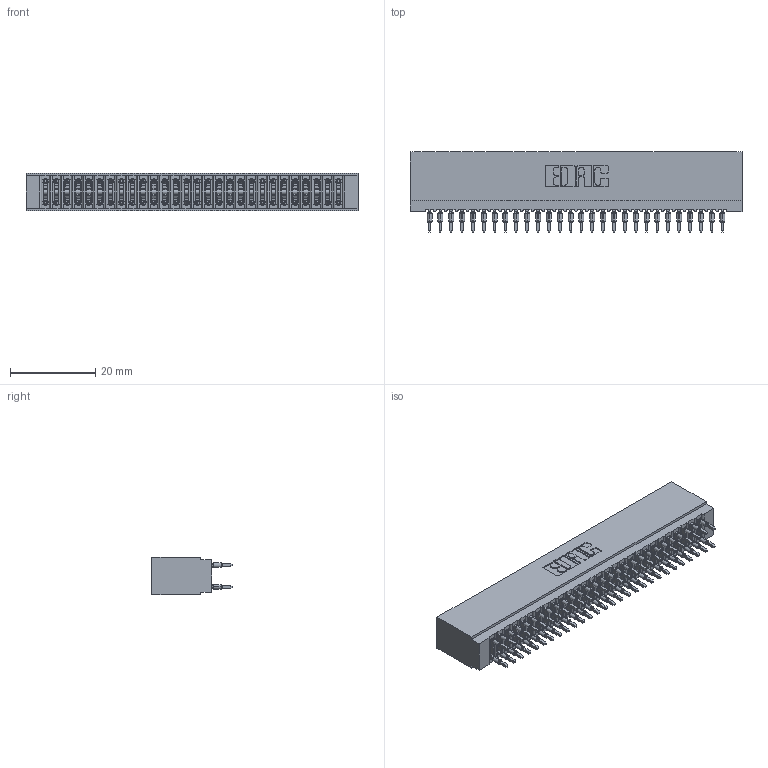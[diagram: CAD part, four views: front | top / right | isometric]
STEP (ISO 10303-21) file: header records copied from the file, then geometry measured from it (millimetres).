
FILE_DESCRIPTION (( 'STEP AP203' ), '1' );
FILE_NAME ('725-056-560-201.STEP', '2026-02-24T18:05:31', ( '' ), ( '' ), 'SwSTEP 2.0', 'SolidWorks 2023', '' );
FILE_SCHEMA (( 'CONFIG_CONTROL_DESIGN' ));
Length unit declared in the file: millimetre
Products named in the file (3): 725-056-560-201; 745-292-001_560; 725 Part_Insulator Option - 01
Assembly tree (57 placements, depth 2):
  725-056-560-201
    725 Part_Insulator Option - 01
    745-292-001_560  x56
Bounding box: 77.72 x 18.8 x 8.89 mm (x, y, z)
Volume: 6441 mm3; surface area: 14187.7 mm2
Topology: 57 solids, 57 shells, 5611 faces, 15346 edges, 9744 vertices
Faces by surface type: plane 2911, cylinder 1244, bspline 1120, torus 336
Entity records: 49337 total; most frequent: CARTESIAN_POINT 9065, ORIENTED_EDGE 8472, DIRECTION 7420, EDGE_CURVE 4236, LINE 3878, VECTOR 3878, VERTEX_POINT 2704, AXIS2_PLACEMENT_3D 1771
